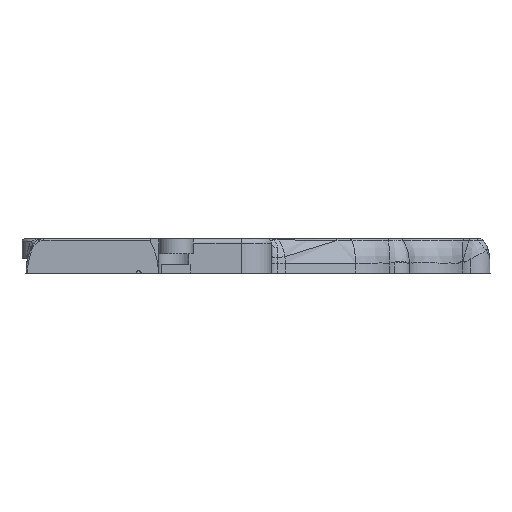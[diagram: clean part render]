
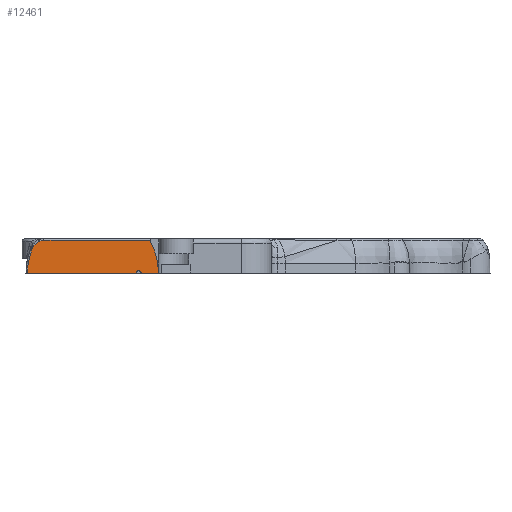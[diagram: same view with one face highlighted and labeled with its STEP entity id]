
A CAD part, left-side view. The second image highlights one B-rep face of the part: STEP entity #12461.
In plain terms, the highlighted planar face has unit normal (-1, 0, 0).
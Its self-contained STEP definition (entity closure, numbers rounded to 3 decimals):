
#40 = CARTESIAN_POINT ( 'NONE',  ( 6.819, 90.254, 10.927 ) ) ;
#334 = ORIENTED_EDGE ( 'NONE', *, *, #3783, .F. ) ;
#655 = CARTESIAN_POINT ( 'NONE',  ( 6.819, 109.529, 11. ) ) ;
#763 = CARTESIAN_POINT ( 'NONE',  ( 6.819, 87.417, 11. ) ) ;
#960 = CARTESIAN_POINT ( 'NONE',  ( 6.819, 129.408, 8.894 ) ) ;
#994 = CARTESIAN_POINT ( 'NONE',  ( 6.819, 125.882, 11. ) ) ;
#1028 = ORIENTED_EDGE ( 'NONE', *, *, #8642, .F. ) ;
#1070 = CARTESIAN_POINT ( 'NONE',  ( 6.819, 129.14, 9.302 ) ) ;
#1080 = ORIENTED_EDGE ( 'NONE', *, *, #13747, .T. ) ;
#1122 = CARTESIAN_POINT ( 'NONE',  ( 6.819, 127.656, 10.522 ) ) ;
#1180 = DIRECTION ( 'NONE',  ( 0., 0., -1. ) ) ;
#1233 = VECTOR ( 'NONE', #4264, 1000. ) ;
#1252 = CARTESIAN_POINT ( 'NONE',  ( 6.819, 129.408, 8.894 ) ) ;
#1536 = VERTEX_POINT ( 'NONE', #5875 ) ;
#1742 = EDGE_LOOP ( 'NONE', ( #1080, #11462, #1028, #3211, #13810, #2777, #10638, #12758, #4818, #334, #2091, #14136 ) ) ;
#2013 = DIRECTION ( 'NONE',  ( 1., 0., 0. ) ) ;
#2091 = ORIENTED_EDGE ( 'NONE', *, *, #11141, .F. ) ;
#2259 = CARTESIAN_POINT ( 'NONE',  ( 6.819, 127.257, 10.69 ) ) ;
#2278 = CARTESIAN_POINT ( 'NONE',  ( 6.819, 109.529, 0. ) ) ;
#2337 = EDGE_CURVE ( 'NONE', #11561, #11812, #13507, .T. ) ;
#2455 = LINE ( 'NONE', #2278, #5532 ) ;
#2615 = DIRECTION ( 'NONE',  ( 1., 0., 0. ) ) ;
#2777 = ORIENTED_EDGE ( 'NONE', *, *, #4461, .F. ) ;
#2938 = CARTESIAN_POINT ( 'NONE',  ( 6.819, 87.679, 0. ) ) ;
#3186 = VERTEX_POINT ( 'NONE', #13336 ) ;
#3201 = CARTESIAN_POINT ( 'NONE',  ( 6.819, 90.254, 10.353 ) ) ;
#3211 = ORIENTED_EDGE ( 'NONE', *, *, #2337, .F. ) ;
#3361 = CARTESIAN_POINT ( 'NONE',  ( 6.819, 129.013, 9.475 ) ) ;
#3733 = CARTESIAN_POINT ( 'NONE',  ( 6.819, 131.379, 0. ) ) ;
#3783 = EDGE_CURVE ( 'NONE', #6617, #13831, #7302, .T. ) ;
#3854 = CARTESIAN_POINT ( 'NONE',  ( 6.819, 129.753, 8.222 ) ) ;
#4212 = DIRECTION ( 'NONE',  ( -1., 0., 0. ) ) ;
#4264 = DIRECTION ( 'NONE',  ( 0., -1., 0. ) ) ;
#4366 = VERTEX_POINT ( 'NONE', #13247 ) ;
#4433 = LINE ( 'NONE', #14765, #1233 ) ;
#4461 = EDGE_CURVE ( 'NONE', #10425, #1536, #5928, .T. ) ;
#4543 = CARTESIAN_POINT ( 'NONE',  ( 6.819, 128.722, 9.795 ) ) ;
#4647 = VERTEX_POINT ( 'NONE', #5386 ) ;
#4725 = CARTESIAN_POINT ( 'NONE',  ( 6.819, 129.311, 9.047 ) ) ;
#4799 = VERTEX_POINT ( 'NONE', #3733 ) ;
#4818 = ORIENTED_EDGE ( 'NONE', *, *, #12992, .F. ) ;
#4980 = B_SPLINE_CURVE_WITH_KNOTS ( 'NONE', 3,
 ( #12599, #1070, #3361, #11450, #4543, #12622, #5709, #13771, #6882, #14926, #8047, #1122, #9192, #2259 ),
 .UNSPECIFIED., .F., .F.,
 ( 4, 2, 2, 2, 2, 2, 4 ),
 ( 0., 0.25, 0.375, 0.438, 0.5, 0.75, 1. ),
 .UNSPECIFIED. ) ;
#5167 = LINE ( 'NONE', #40, #10945 ) ;
#5386 = CARTESIAN_POINT ( 'NONE',  ( 6.819, 95.159, 0. ) ) ;
#5500 = AXIS2_PLACEMENT_3D ( 'NONE', #8943, #2013, #10106 ) ;
#5532 = VECTOR ( 'NONE', #9208, 1000. ) ;
#5587 = CARTESIAN_POINT ( 'NONE',  ( 6.819, 126.817, 10.865 ) ) ;
#5709 = CARTESIAN_POINT ( 'NONE',  ( 6.819, 128.561, 9.942 ) ) ;
#5875 = CARTESIAN_POINT ( 'NONE',  ( 6.819, 90.254, 11. ) ) ;
#5928 = LINE ( 'NONE', #655, #8986 ) ;
#6165 = CARTESIAN_POINT ( 'NONE',  ( 6.819, 129.408, 8.894 ) ) ;
#6547 =( BOUNDED_CURVE ( )  B_SPLINE_CURVE ( 3, ( #8304, #8492, #10794, #3854 ),
 .UNSPECIFIED., .F., .F. ) 
 B_SPLINE_CURVE_WITH_KNOTS ( ( 4, 4 ),
 ( 0., 1. ),
 .UNSPECIFIED. ) 
 CURVE ( )  GEOMETRIC_REPRESENTATION_ITEM ( )  RATIONAL_B_SPLINE_CURVE ( ( 0.957, 0.944, 0.944, 0.957 ) ) 
 REPRESENTATION_ITEM ( '' )  );
#6617 = VERTEX_POINT ( 'NONE', #11532 ) ;
#6713 = CARTESIAN_POINT ( 'NONE',  ( 6.819, 129.753, 8.222 ) ) ;
#6788 = VERTEX_POINT ( 'NONE', #14187 ) ;
#6857 = DIRECTION ( 'NONE',  ( 1., 0., 0. ) ) ;
#6882 = CARTESIAN_POINT ( 'NONE',  ( 6.819, 128.435, 10.046 ) ) ;
#7302 =( BOUNDED_CURVE ( )  B_SPLINE_CURVE ( 3, ( #6713, #14772, #7890, #960 ),
 .UNSPECIFIED., .F., .T. ) 
 B_SPLINE_CURVE_WITH_KNOTS ( ( 4, 4 ),
 ( 0., 1. ),
 .UNSPECIFIED. ) 
 CURVE ( )  GEOMETRIC_REPRESENTATION_ITEM ( )  RATIONAL_B_SPLINE_CURVE ( ( 0.957, 0.954, 0.954, 0.957 ) ) 
 REPRESENTATION_ITEM ( '' )  );
#7314 = EDGE_CURVE ( 'NONE', #4799, #4647, #4433, .T. ) ;
#7395 = EDGE_CURVE ( 'NONE', #3186, #10425, #11077, .T. ) ;
#7568 = AXIS2_PLACEMENT_3D ( 'NONE', #9548, #2615, #10695 ) ;
#7704 = CIRCLE ( 'NONE', #7568, 0.844 ) ;
#7804 = CARTESIAN_POINT ( 'NONE',  ( 6.819, 94.315, 0.844 ) ) ;
#7890 = CARTESIAN_POINT ( 'NONE',  ( 6.819, 129.541, 8.68 ) ) ;
#7891 = AXIS2_PLACEMENT_3D ( 'NONE', #13745, #6857, #14894 ) ;
#7931 = CARTESIAN_POINT ( 'NONE',  ( 6.819, 126.355, 10.969 ) ) ;
#8047 = CARTESIAN_POINT ( 'NONE',  ( 6.819, 128.037, 10.323 ) ) ;
#8304 = CARTESIAN_POINT ( 'NONE',  ( 6.819, 131.379, 0. ) ) ;
#8492 = CARTESIAN_POINT ( 'NONE',  ( 6.819, 131.379, 2.83 ) ) ;
#8642 = EDGE_CURVE ( 'NONE', #11812, #4366, #2455, .T. ) ;
#8661 = EDGE_CURVE ( 'NONE', #1536, #11561, #5167, .T. ) ;
#8719 = DIRECTION ( 'NONE',  ( 0., -1., 0. ) ) ;
#8836 = PLANE ( 'NONE',  #9952 ) ;
#8943 = CARTESIAN_POINT ( 'NONE',  ( 6.819, 94.315, 0. ) ) ;
#8986 = VECTOR ( 'NONE', #8719, 1000. ) ;
#9192 = CARTESIAN_POINT ( 'NONE',  ( 6.819, 127.458, 10.61 ) ) ;
#9208 = DIRECTION ( 'NONE',  ( 0., 1., 0. ) ) ;
#9316 = CARTESIAN_POINT ( 'NONE',  ( 6.819, 129.36, 8.97 ) ) ;
#9548 = CARTESIAN_POINT ( 'NONE',  ( 6.819, 94.315, 0. ) ) ;
#9952 = AXIS2_PLACEMENT_3D ( 'NONE', #763, #4212, #12306 ) ;
#10106 = DIRECTION ( 'NONE',  ( 0., 0., -1. ) ) ;
#10425 = VERTEX_POINT ( 'NONE', #11339 ) ;
#10638 = ORIENTED_EDGE ( 'NONE', *, *, #7395, .F. ) ;
#10695 = DIRECTION ( 'NONE',  ( 0., 0., -1. ) ) ;
#10794 = CARTESIAN_POINT ( 'NONE',  ( 6.819, 130.83, 5.606 ) ) ;
#10870 = EDGE_CURVE ( 'NONE', #6788, #3186, #4980, .T. ) ;
#10945 = VECTOR ( 'NONE', #1180, 1000. ) ;
#11077 =( BOUNDED_CURVE ( )  B_SPLINE_CURVE ( 3, ( #13648, #5587, #7931, #994 ),
 .UNSPECIFIED., .F., .T. ) 
 B_SPLINE_CURVE_WITH_KNOTS ( ( 4, 4 ),
 ( 0., 1. ),
 .UNSPECIFIED. ) 
 CURVE ( )  GEOMETRIC_REPRESENTATION_ITEM ( )  RATIONAL_B_SPLINE_CURVE ( ( 0.957, 0.949, 0.948, 0.956 ) ) 
 REPRESENTATION_ITEM ( '' )  );
#11141 = EDGE_CURVE ( 'NONE', #4799, #6617, #6547, .T. ) ;
#11339 = CARTESIAN_POINT ( 'NONE',  ( 6.819, 125.882, 11. ) ) ;
#11450 = CARTESIAN_POINT ( 'NONE',  ( 6.819, 128.798, 9.717 ) ) ;
#11462 = ORIENTED_EDGE ( 'NONE', *, *, #13255, .T. ) ;
#11532 = CARTESIAN_POINT ( 'NONE',  ( 6.819, 129.753, 8.222 ) ) ;
#11561 = VERTEX_POINT ( 'NONE', #3201 ) ;
#11812 = VERTEX_POINT ( 'NONE', #2938 ) ;
#12306 = DIRECTION ( 'NONE',  ( 0., 0., -1. ) ) ;
#12461 = ADVANCED_FACE ( 'NONE', ( #14141 ), #8836, .T. ) ;
#12599 = CARTESIAN_POINT ( 'NONE',  ( 6.819, 129.26, 9.122 ) ) ;
#12622 = CARTESIAN_POINT ( 'NONE',  ( 6.819, 128.602, 9.906 ) ) ;
#12758 = ORIENTED_EDGE ( 'NONE', *, *, #10870, .F. ) ;
#12802 = CARTESIAN_POINT ( 'NONE',  ( 6.819, 129.26, 9.122 ) ) ;
#12992 = EDGE_CURVE ( 'NONE', #13831, #6788, #14378, .T. ) ;
#13247 = CARTESIAN_POINT ( 'NONE',  ( 6.819, 93.471, 0. ) ) ;
#13255 = EDGE_CURVE ( 'NONE', #13260, #4366, #13290, .T. ) ;
#13260 = VERTEX_POINT ( 'NONE', #7804 ) ;
#13290 = CIRCLE ( 'NONE', #5500, 0.844 ) ;
#13336 = CARTESIAN_POINT ( 'NONE',  ( 6.819, 127.257, 10.69 ) ) ;
#13507 = CIRCLE ( 'NONE', #7891, 22.1 ) ;
#13648 = CARTESIAN_POINT ( 'NONE',  ( 6.819, 127.257, 10.69 ) ) ;
#13745 = CARTESIAN_POINT ( 'NONE',  ( 6.819, 109.779, 0. ) ) ;
#13747 = EDGE_CURVE ( 'NONE', #4647, #13260, #7704, .T. ) ;
#13771 = CARTESIAN_POINT ( 'NONE',  ( 6.819, 128.478, 10.013 ) ) ;
#13810 = ORIENTED_EDGE ( 'NONE', *, *, #8661, .F. ) ;
#13831 = VERTEX_POINT ( 'NONE', #6165 ) ;
#14136 = ORIENTED_EDGE ( 'NONE', *, *, #7314, .T. ) ;
#14141 = FACE_OUTER_BOUND ( 'NONE', #1742, .T. ) ;
#14187 = CARTESIAN_POINT ( 'NONE',  ( 6.819, 129.26, 9.122 ) ) ;
#14378 = B_SPLINE_CURVE_WITH_KNOTS ( 'NONE', 3,
 ( #1252, #9316, #4725, #12802 ),
 .UNSPECIFIED., .F., .F.,
 ( 4, 4 ),
 ( 0., 1. ),
 .UNSPECIFIED. ) ;
#14765 = CARTESIAN_POINT ( 'NONE',  ( 6.819, 54.009, 0. ) ) ;
#14772 = CARTESIAN_POINT ( 'NONE',  ( 6.819, 129.657, 8.455 ) ) ;
#14894 = DIRECTION ( 'NONE',  ( 0., 0., -1. ) ) ;
#14926 = CARTESIAN_POINT ( 'NONE',  ( 6.819, 128.22, 10.21 ) ) ;
